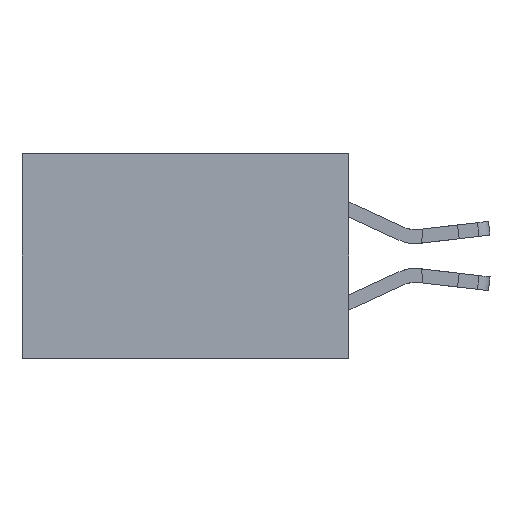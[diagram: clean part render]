
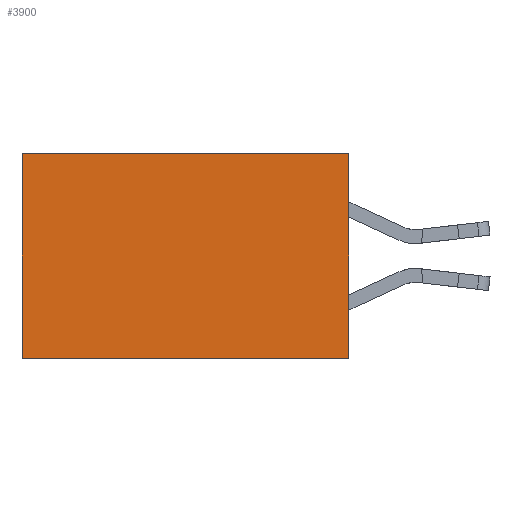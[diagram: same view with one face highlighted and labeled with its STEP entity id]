
A CAD part, left-side view. The second image highlights one B-rep face of the part: STEP entity #3900.
In plain terms, the highlighted planar face has unit normal (-1, 0, 0).
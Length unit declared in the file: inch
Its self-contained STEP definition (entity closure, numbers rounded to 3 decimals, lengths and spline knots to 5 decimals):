
#259 = EDGE_LOOP ( 'NONE', ( #7449, #6047, #9755, #8677 ) ) ;
#530 = PLANE ( 'NONE',  #11958 ) ;
#1349 = CARTESIAN_POINT ( 'NONE',  ( 0.277, 0., -0.37 ) ) ;
#1518 = CARTESIAN_POINT ( 'NONE',  ( 0.277, 0., -0.37 ) ) ;
#1867 = CARTESIAN_POINT ( 'NONE',  ( 0.277, 0., -0.37 ) ) ;
#1924 = DIRECTION ( 'NONE',  ( 0., 0., -1. ) ) ;
#1979 = VERTEX_POINT ( 'NONE', #12583 ) ;
#2655 = DIRECTION ( 'NONE',  ( 0., 1., 0. ) ) ;
#3003 = VERTEX_POINT ( 'NONE', #12676 ) ;
#3198 = CARTESIAN_POINT ( 'NONE',  ( 0.277, 0., -0.37 ) ) ;
#3717 = DIRECTION ( 'NONE',  ( 0., 0., -1. ) ) ;
#3900 = ADVANCED_FACE ( 'NONE', ( #6205 ), #530, .F. ) ;
#4352 = CARTESIAN_POINT ( 'NONE',  ( 0.277, 0., 0. ) ) ;
#4930 = EDGE_CURVE ( 'NONE', #10784, #3003, #9668, .T. ) ;
#5070 = VECTOR ( 'NONE', #2655, 39.37008 ) ;
#5427 = VERTEX_POINT ( 'NONE', #1518 ) ;
#6047 = ORIENTED_EDGE ( 'NONE', *, *, #7971, .F. ) ;
#6205 = FACE_OUTER_BOUND ( 'NONE', #259, .T. ) ;
#7081 = EDGE_CURVE ( 'NONE', #3003, #1979, #9202, .T. ) ;
#7304 = CARTESIAN_POINT ( 'NONE',  ( 0.277, 0.59, -0.37 ) ) ;
#7449 = ORIENTED_EDGE ( 'NONE', *, *, #7081, .T. ) ;
#7568 = EDGE_CURVE ( 'NONE', #10784, #5427, #10947, .T. ) ;
#7971 = EDGE_CURVE ( 'NONE', #5427, #1979, #14937, .T. ) ;
#8419 = VECTOR ( 'NONE', #11071, 39.37008 ) ;
#8677 = ORIENTED_EDGE ( 'NONE', *, *, #4930, .T. ) ;
#9202 = LINE ( 'NONE', #7304, #8419 ) ;
#9668 = LINE ( 'NONE', #11914, #15772 ) ;
#9755 = ORIENTED_EDGE ( 'NONE', *, *, #7568, .F. ) ;
#10784 = VERTEX_POINT ( 'NONE', #4352 ) ;
#10947 = LINE ( 'NONE', #1867, #14200 ) ;
#11071 = DIRECTION ( 'NONE',  ( 0., 0., -1. ) ) ;
#11373 = DIRECTION ( 'NONE',  ( 1., 0., 0. ) ) ;
#11817 = DIRECTION ( 'NONE',  ( 0., 1., 0. ) ) ;
#11914 = CARTESIAN_POINT ( 'NONE',  ( 0.277, 0., 0. ) ) ;
#11958 = AXIS2_PLACEMENT_3D ( 'NONE', #3198, #11373, #3717 ) ;
#12583 = CARTESIAN_POINT ( 'NONE',  ( 0.277, 0.59, -0.37 ) ) ;
#12676 = CARTESIAN_POINT ( 'NONE',  ( 0.277, 0.59, 0. ) ) ;
#14200 = VECTOR ( 'NONE', #1924, 39.37008 ) ;
#14937 = LINE ( 'NONE', #1349, #5070 ) ;
#15772 = VECTOR ( 'NONE', #11817, 39.37008 ) ;
